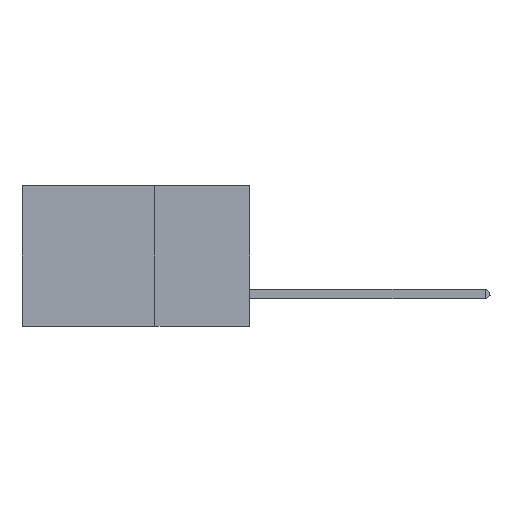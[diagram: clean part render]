
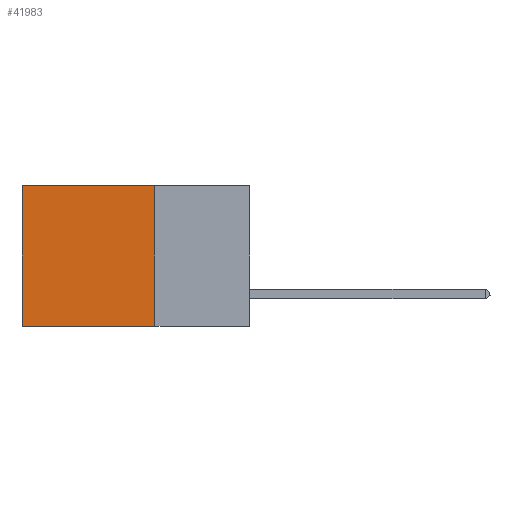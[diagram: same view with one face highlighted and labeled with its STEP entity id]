
A CAD part, left-side view. The second image highlights one B-rep face of the part: STEP entity #41983.
In plain terms, the highlighted planar face has unit normal (-1, 0, 0).
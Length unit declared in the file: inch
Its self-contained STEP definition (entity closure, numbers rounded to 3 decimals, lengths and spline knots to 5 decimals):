
#1307 = DIRECTION ( 'NONE',  ( 0., 0., -1. ) ) ;
#3197 = DIRECTION ( 'NONE',  ( 1., 0., 0. ) ) ;
#4480 = VECTOR ( 'NONE', #25212, 39.37008 ) ;
#5670 = LINE ( 'NONE', #48892, #37675 ) ;
#9088 = EDGE_LOOP ( 'NONE', ( #49714, #44387, #30390, #35298 ) ) ;
#10413 = VERTEX_POINT ( 'NONE', #25279 ) ;
#14789 = LINE ( 'NONE', #24518, #4480 ) ;
#15823 = EDGE_CURVE ( 'NONE', #10413, #48629, #14789, .T. ) ;
#16213 = CARTESIAN_POINT ( 'NONE',  ( 0.2875, 0.6, 0. ) ) ;
#17504 = VERTEX_POINT ( 'NONE', #19973 ) ;
#19973 = CARTESIAN_POINT ( 'NONE',  ( 0.2875, 0.6, 0. ) ) ;
#20487 = VERTEX_POINT ( 'NONE', #49896 ) ;
#22494 = PLANE ( 'NONE',  #48529 ) ;
#24221 = VECTOR ( 'NONE', #1307, 39.37008 ) ;
#24518 = CARTESIAN_POINT ( 'NONE',  ( 0.2875, 0.25, 0. ) ) ;
#24684 = LINE ( 'NONE', #44693, #44678 ) ;
#25212 = DIRECTION ( 'NONE',  ( 0., 0., -1. ) ) ;
#25279 = CARTESIAN_POINT ( 'NONE',  ( 0.2875, 0.25, 0. ) ) ;
#25911 = EDGE_CURVE ( 'NONE', #10413, #17504, #5670, .T. ) ;
#27297 = EDGE_CURVE ( 'NONE', #17504, #20487, #33286, .T. ) ;
#30255 = DIRECTION ( 'NONE',  ( 0., 0., -1. ) ) ;
#30390 = ORIENTED_EDGE ( 'NONE', *, *, #15823, .F. ) ;
#33286 = LINE ( 'NONE', #16213, #24221 ) ;
#34397 = CARTESIAN_POINT ( 'NONE',  ( 0.2875, 0.25, -0.37 ) ) ;
#35298 = ORIENTED_EDGE ( 'NONE', *, *, #25911, .T. ) ;
#37675 = VECTOR ( 'NONE', #40929, 39.37008 ) ;
#40929 = DIRECTION ( 'NONE',  ( 0., 1., 0. ) ) ;
#41840 = EDGE_CURVE ( 'NONE', #48629, #20487, #24684, .T. ) ;
#41983 = ADVANCED_FACE ( 'NONE', ( #46460 ), #22494, .F. ) ;
#44387 = ORIENTED_EDGE ( 'NONE', *, *, #41840, .F. ) ;
#44678 = VECTOR ( 'NONE', #48744, 39.37008 ) ;
#44693 = CARTESIAN_POINT ( 'NONE',  ( 0.2875, 0.25, -0.37 ) ) ;
#46460 = FACE_OUTER_BOUND ( 'NONE', #9088, .T. ) ;
#48529 = AXIS2_PLACEMENT_3D ( 'NONE', #49581, #3197, #30255 ) ;
#48629 = VERTEX_POINT ( 'NONE', #34397 ) ;
#48744 = DIRECTION ( 'NONE',  ( 0., 1., 0. ) ) ;
#48892 = CARTESIAN_POINT ( 'NONE',  ( 0.2875, 0.25, 0. ) ) ;
#49581 = CARTESIAN_POINT ( 'NONE',  ( 0.2875, 0.25, 0. ) ) ;
#49714 = ORIENTED_EDGE ( 'NONE', *, *, #27297, .T. ) ;
#49896 = CARTESIAN_POINT ( 'NONE',  ( 0.2875, 0.6, -0.37 ) ) ;
